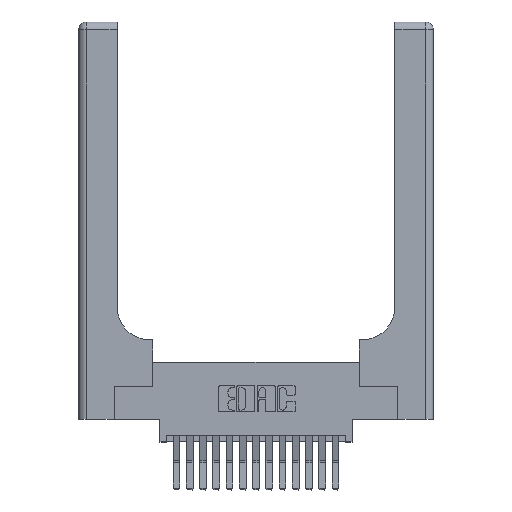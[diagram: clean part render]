
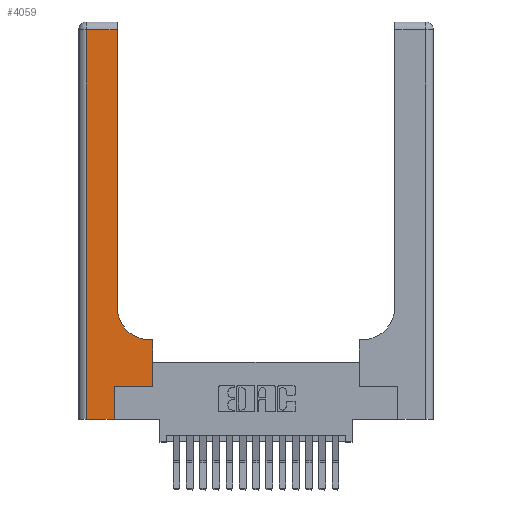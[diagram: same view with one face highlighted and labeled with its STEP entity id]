
A CAD part, top view. The second image highlights one B-rep face of the part: STEP entity #4059.
In plain terms, the highlighted planar face has unit normal (0, 0, 1).
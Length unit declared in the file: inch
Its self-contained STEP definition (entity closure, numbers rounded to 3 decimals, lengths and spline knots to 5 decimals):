
#253 = VERTEX_POINT ( 'NONE', #7283 ) ;
#322 = VECTOR ( 'NONE', #15809, 39.37008 ) ;
#392 = DIRECTION ( 'NONE',  ( 0., 0., -1. ) ) ;
#1385 = CARTESIAN_POINT ( 'NONE',  ( 0.2915, 0.85, 0.37 ) ) ;
#1509 = VECTOR ( 'NONE', #1956, 39.37008 ) ;
#1740 = LINE ( 'NONE', #6136, #9245 ) ;
#1751 = LINE ( 'NONE', #10924, #1509 ) ;
#1956 = DIRECTION ( 'NONE',  ( 1., 0., 0. ) ) ;
#2178 = EDGE_CURVE ( 'NONE', #4275, #5340, #17939, .T. ) ;
#2236 = CARTESIAN_POINT ( 'NONE',  ( 0.269, 0., 0.37 ) ) ;
#2979 = DIRECTION ( 'NONE',  ( 1., 0., 0. ) ) ;
#3095 = DIRECTION ( 'NONE',  ( 0., 1., 0. ) ) ;
#3473 = LINE ( 'NONE', #2236, #15464 ) ;
#3722 = LINE ( 'NONE', #18532, #10292 ) ;
#3936 = EDGE_CURVE ( 'NONE', #253, #14588, #3722, .T. ) ;
#4059 = ADVANCED_FACE ( 'NONE', ( #11225 ), #7445, .F. ) ;
#4148 = ORIENTED_EDGE ( 'NONE', *, *, #2178, .T. ) ;
#4275 = VERTEX_POINT ( 'NONE', #9659 ) ;
#4334 = LINE ( 'NONE', #8145, #322 ) ;
#4610 = ORIENTED_EDGE ( 'NONE', *, *, #8622, .T. ) ;
#4629 = DIRECTION ( 'NONE',  ( -1., 0., 0. ) ) ;
#4950 = LINE ( 'NONE', #18676, #15516 ) ;
#4958 = EDGE_CURVE ( 'NONE', #12324, #19487, #3473, .T. ) ;
#5340 = VERTEX_POINT ( 'NONE', #14662 ) ;
#5726 = LINE ( 'NONE', #15316, #10409 ) ;
#5884 = ORIENTED_EDGE ( 'NONE', *, *, #19048, .T. ) ;
#6136 = CARTESIAN_POINT ( 'NONE',  ( 0., 0., 0.37 ) ) ;
#6321 = VERTEX_POINT ( 'NONE', #1385 ) ;
#6811 = EDGE_LOOP ( 'NONE', ( #5884, #4148, #9725, #16362, #7066, #4610, #18435, #13937, #7522 ) ) ;
#7066 = ORIENTED_EDGE ( 'NONE', *, *, #4958, .T. ) ;
#7283 = CARTESIAN_POINT ( 'NONE',  ( 0.5585, 0.25, 0.37 ) ) ;
#7445 = PLANE ( 'NONE',  #12725 ) ;
#7522 = ORIENTED_EDGE ( 'NONE', *, *, #18579, .T. ) ;
#7833 = DIRECTION ( 'NONE',  ( 0., 0., -1. ) ) ;
#8104 = DIRECTION ( 'NONE',  ( 0., 1., 0. ) ) ;
#8145 = CARTESIAN_POINT ( 'NONE',  ( 0.2915, 0.6, 0.37 ) ) ;
#8622 = EDGE_CURVE ( 'NONE', #19487, #253, #1751, .T. ) ;
#8652 = CARTESIAN_POINT ( 'NONE',  ( 0.5415, 0.6, 0.37 ) ) ;
#8797 = CIRCLE ( 'NONE', #18831, 0.25 ) ;
#8970 = CARTESIAN_POINT ( 'NONE',  ( 0., 3., 0.37 ) ) ;
#9245 = VECTOR ( 'NONE', #2979, 39.37008 ) ;
#9551 = CARTESIAN_POINT ( 'NONE',  ( 0.06, 0., 0.37 ) ) ;
#9659 = CARTESIAN_POINT ( 'NONE',  ( 0.2915, 2.94, 0.37 ) ) ;
#9725 = ORIENTED_EDGE ( 'NONE', *, *, #16996, .T. ) ;
#10292 = VECTOR ( 'NONE', #3095, 39.37008 ) ;
#10409 = VECTOR ( 'NONE', #8104, 39.37008 ) ;
#10910 = DIRECTION ( 'NONE',  ( 1., 0., 0. ) ) ;
#10924 = CARTESIAN_POINT ( 'NONE',  ( 0.269, 0.25, 0.37 ) ) ;
#11225 = FACE_OUTER_BOUND ( 'NONE', #6811, .T. ) ;
#11839 = CARTESIAN_POINT ( 'NONE',  ( 0.269, 0.25, 0.37 ) ) ;
#12019 = VECTOR ( 'NONE', #15533, 39.37008 ) ;
#12324 = VERTEX_POINT ( 'NONE', #12459 ) ;
#12447 = CARTESIAN_POINT ( 'NONE',  ( 0., 2.94, 0.37 ) ) ;
#12453 = DIRECTION ( 'NONE',  ( 0., 1., 0. ) ) ;
#12459 = CARTESIAN_POINT ( 'NONE',  ( 0.269, 0., 0.37 ) ) ;
#12725 = AXIS2_PLACEMENT_3D ( 'NONE', #8970, #7833, #4629 ) ;
#12791 = DIRECTION ( 'NONE',  ( 0., -1., 0. ) ) ;
#13937 = ORIENTED_EDGE ( 'NONE', *, *, #18626, .T. ) ;
#14347 = CARTESIAN_POINT ( 'NONE',  ( 0.5585, 0.6, 0.37 ) ) ;
#14588 = VERTEX_POINT ( 'NONE', #14347 ) ;
#14662 = CARTESIAN_POINT ( 'NONE',  ( 0.06, 2.94, 0.37 ) ) ;
#15316 = CARTESIAN_POINT ( 'NONE',  ( 0.2915, 3., 0.37 ) ) ;
#15431 = CARTESIAN_POINT ( 'NONE',  ( 0.5415, 0.85, 0.37 ) ) ;
#15464 = VECTOR ( 'NONE', #12453, 39.37008 ) ;
#15516 = VECTOR ( 'NONE', #12791, 39.37008 ) ;
#15533 = DIRECTION ( 'NONE',  ( -1., 0., 0. ) ) ;
#15809 = DIRECTION ( 'NONE',  ( -1., 0., 0. ) ) ;
#16053 = EDGE_CURVE ( 'NONE', #17436, #12324, #1740, .T. ) ;
#16362 = ORIENTED_EDGE ( 'NONE', *, *, #16053, .T. ) ;
#16569 = VERTEX_POINT ( 'NONE', #8652 ) ;
#16996 = EDGE_CURVE ( 'NONE', #5340, #17436, #4950, .T. ) ;
#17436 = VERTEX_POINT ( 'NONE', #9551 ) ;
#17939 = LINE ( 'NONE', #12447, #12019 ) ;
#18435 = ORIENTED_EDGE ( 'NONE', *, *, #3936, .T. ) ;
#18532 = CARTESIAN_POINT ( 'NONE',  ( 0.5585, 0.25, 0.37 ) ) ;
#18579 = EDGE_CURVE ( 'NONE', #16569, #6321, #8797, .T. ) ;
#18626 = EDGE_CURVE ( 'NONE', #14588, #16569, #4334, .T. ) ;
#18676 = CARTESIAN_POINT ( 'NONE',  ( 0.06, 3., 0.37 ) ) ;
#18831 = AXIS2_PLACEMENT_3D ( 'NONE', #15431, #392, #10910 ) ;
#19048 = EDGE_CURVE ( 'NONE', #6321, #4275, #5726, .T. ) ;
#19487 = VERTEX_POINT ( 'NONE', #11839 ) ;
